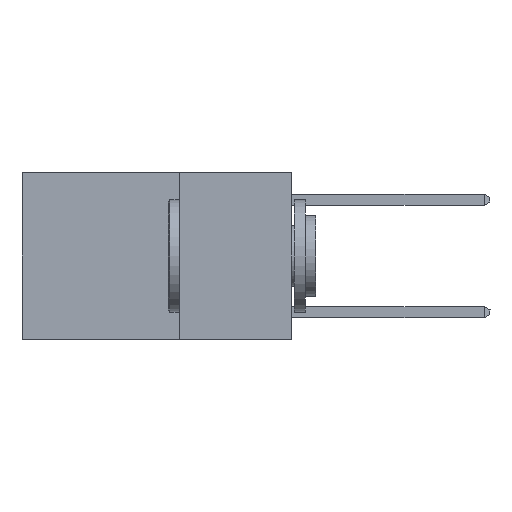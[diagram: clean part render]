
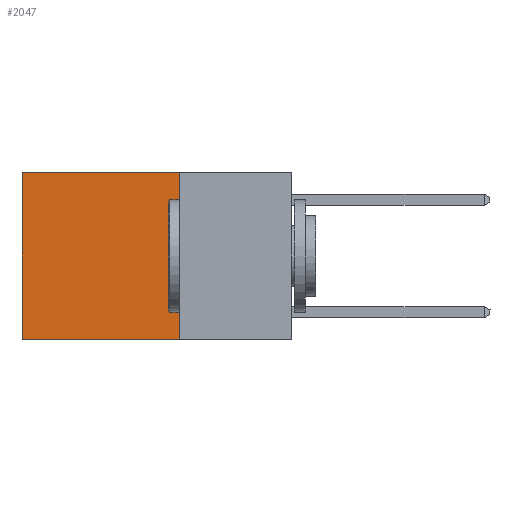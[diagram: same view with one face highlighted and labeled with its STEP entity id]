
A CAD part, left-side view. The second image highlights one B-rep face of the part: STEP entity #2047.
In plain terms, the highlighted planar face has unit normal (-1, 0, 0).
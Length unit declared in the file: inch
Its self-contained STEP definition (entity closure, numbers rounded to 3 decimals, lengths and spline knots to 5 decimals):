
#54 = VECTOR ( 'NONE', #10496, 39.37008 ) ;
#246 = DIRECTION ( 'NONE',  ( 0., 0., -1. ) ) ;
#478 = LINE ( 'NONE', #15019, #4913 ) ;
#553 = VECTOR ( 'NONE', #22624, 39.37008 ) ;
#887 = CARTESIAN_POINT ( 'NONE',  ( 0.2625, 0.25, 0. ) ) ;
#1563 = VERTEX_POINT ( 'NONE', #8768 ) ;
#2047 = ADVANCED_FACE ( 'NONE', ( #21589 ), #3738, .F. ) ;
#3444 = EDGE_LOOP ( 'NONE', ( #3952, #14750, #13091, #6254 ) ) ;
#3685 = DIRECTION ( 'NONE',  ( 0., 0., -1. ) ) ;
#3716 = DIRECTION ( 'NONE',  ( 1., 0., 0. ) ) ;
#3738 = PLANE ( 'NONE',  #19864 ) ;
#3795 = CARTESIAN_POINT ( 'NONE',  ( 0.2625, 0.25, 0. ) ) ;
#3952 = ORIENTED_EDGE ( 'NONE', *, *, #9390, .T. ) ;
#4887 = EDGE_CURVE ( 'NONE', #1563, #17210, #9673, .T. ) ;
#4913 = VECTOR ( 'NONE', #246, 39.37008 ) ;
#6254 = ORIENTED_EDGE ( 'NONE', *, *, #14180, .T. ) ;
#8613 = CARTESIAN_POINT ( 'NONE',  ( 0.2625, 0.6, 0. ) ) ;
#8768 = CARTESIAN_POINT ( 'NONE',  ( 0.2625, 0.25, -0.37 ) ) ;
#9390 = EDGE_CURVE ( 'NONE', #9810, #17210, #14882, .T. ) ;
#9673 = LINE ( 'NONE', #10054, #23212 ) ;
#9810 = VERTEX_POINT ( 'NONE', #20419 ) ;
#10054 = CARTESIAN_POINT ( 'NONE',  ( 0.2625, 0.25, -0.37 ) ) ;
#10496 = DIRECTION ( 'NONE',  ( 0., 0., -1. ) ) ;
#10572 = LINE ( 'NONE', #20937, #553 ) ;
#13091 = ORIENTED_EDGE ( 'NONE', *, *, #22709, .F. ) ;
#13677 = VERTEX_POINT ( 'NONE', #887 ) ;
#14180 = EDGE_CURVE ( 'NONE', #13677, #9810, #10572, .T. ) ;
#14750 = ORIENTED_EDGE ( 'NONE', *, *, #4887, .F. ) ;
#14882 = LINE ( 'NONE', #8613, #54 ) ;
#15019 = CARTESIAN_POINT ( 'NONE',  ( 0.2625, 0.25, 0. ) ) ;
#17210 = VERTEX_POINT ( 'NONE', #21698 ) ;
#19864 = AXIS2_PLACEMENT_3D ( 'NONE', #3795, #3716, #3685 ) ;
#20419 = CARTESIAN_POINT ( 'NONE',  ( 0.2625, 0.6, 0. ) ) ;
#20937 = CARTESIAN_POINT ( 'NONE',  ( 0.2625, 0.25, 0. ) ) ;
#21589 = FACE_OUTER_BOUND ( 'NONE', #3444, .T. ) ;
#21698 = CARTESIAN_POINT ( 'NONE',  ( 0.2625, 0.6, -0.37 ) ) ;
#22451 = DIRECTION ( 'NONE',  ( 0., 1., 0. ) ) ;
#22624 = DIRECTION ( 'NONE',  ( 0., 1., 0. ) ) ;
#22709 = EDGE_CURVE ( 'NONE', #13677, #1563, #478, .T. ) ;
#23212 = VECTOR ( 'NONE', #22451, 39.37008 ) ;
